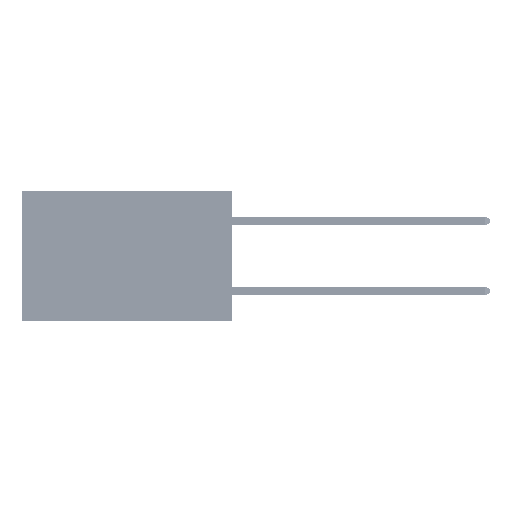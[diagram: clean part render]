
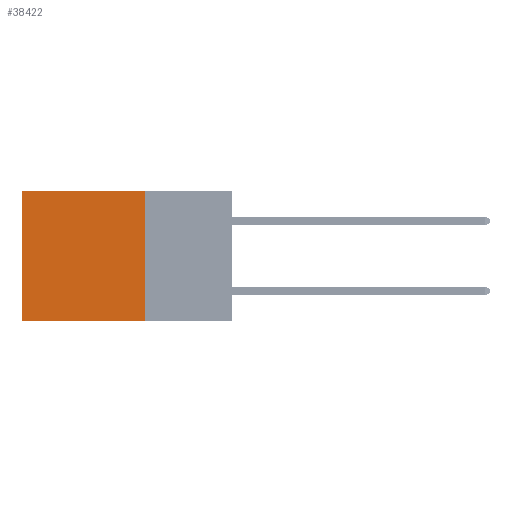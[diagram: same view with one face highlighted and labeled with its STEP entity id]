
A CAD part, left-side view. The second image highlights one B-rep face of the part: STEP entity #38422.
In plain terms, the highlighted planar face has unit normal (-1, 0, 0).
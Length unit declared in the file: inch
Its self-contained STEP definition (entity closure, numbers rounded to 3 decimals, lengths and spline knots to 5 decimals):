
#2273 = CARTESIAN_POINT ( 'NONE',  ( 0.2875, 0.25, -0.37 ) ) ;
#2553 = CARTESIAN_POINT ( 'NONE',  ( 0.2875, 0.6, -0.37 ) ) ;
#2675 = PLANE ( 'NONE',  #5106 ) ;
#3037 = VERTEX_POINT ( 'NONE', #2553 ) ;
#5106 = AXIS2_PLACEMENT_3D ( 'NONE', #10620, #38117, #14596 ) ;
#5762 = FACE_OUTER_BOUND ( 'NONE', #46328, .T. ) ;
#6406 = VECTOR ( 'NONE', #40510, 39.37008 ) ;
#7639 = LINE ( 'NONE', #8894, #6406 ) ;
#8161 = EDGE_CURVE ( 'NONE', #40035, #40743, #30784, .T. ) ;
#8890 = ORIENTED_EDGE ( 'NONE', *, *, #32610, .F. ) ;
#8894 = CARTESIAN_POINT ( 'NONE',  ( 0.2875, 0.6, 0. ) ) ;
#9358 = LINE ( 'NONE', #11701, #27846 ) ;
#10620 = CARTESIAN_POINT ( 'NONE',  ( 0.2875, 0.25, 0. ) ) ;
#11701 = CARTESIAN_POINT ( 'NONE',  ( 0.2875, 0.25, 0. ) ) ;
#12094 = EDGE_CURVE ( 'NONE', #24547, #3037, #33833, .T. ) ;
#14596 = DIRECTION ( 'NONE',  ( 0., 0., -1. ) ) ;
#18490 = CARTESIAN_POINT ( 'NONE',  ( 0.2875, 0.25, 0. ) ) ;
#19966 = ORIENTED_EDGE ( 'NONE', *, *, #8161, .T. ) ;
#20305 = VECTOR ( 'NONE', #20555, 39.37008 ) ;
#20555 = DIRECTION ( 'NONE',  ( 0., 1., 0. ) ) ;
#20885 = VECTOR ( 'NONE', #37561, 39.37008 ) ;
#24547 = VERTEX_POINT ( 'NONE', #40004 ) ;
#25428 = ORIENTED_EDGE ( 'NONE', *, *, #12094, .F. ) ;
#27353 = CARTESIAN_POINT ( 'NONE',  ( 0.2875, 0.6, 0. ) ) ;
#27846 = VECTOR ( 'NONE', #47047, 39.37008 ) ;
#30784 = LINE ( 'NONE', #44053, #20305 ) ;
#32610 = EDGE_CURVE ( 'NONE', #40035, #24547, #9358, .T. ) ;
#33833 = LINE ( 'NONE', #2273, #20885 ) ;
#37561 = DIRECTION ( 'NONE',  ( 0., 1., 0. ) ) ;
#38117 = DIRECTION ( 'NONE',  ( 1., 0., 0. ) ) ;
#38152 = EDGE_CURVE ( 'NONE', #40743, #3037, #7639, .T. ) ;
#38422 = ADVANCED_FACE ( 'NONE', ( #5762 ), #2675, .F. ) ;
#40004 = CARTESIAN_POINT ( 'NONE',  ( 0.2875, 0.25, -0.37 ) ) ;
#40035 = VERTEX_POINT ( 'NONE', #18490 ) ;
#40510 = DIRECTION ( 'NONE',  ( 0., 0., -1. ) ) ;
#40743 = VERTEX_POINT ( 'NONE', #27353 ) ;
#44053 = CARTESIAN_POINT ( 'NONE',  ( 0.2875, 0.25, 0. ) ) ;
#46328 = EDGE_LOOP ( 'NONE', ( #46437, #25428, #8890, #19966 ) ) ;
#46437 = ORIENTED_EDGE ( 'NONE', *, *, #38152, .T. ) ;
#47047 = DIRECTION ( 'NONE',  ( 0., 0., -1. ) ) ;
